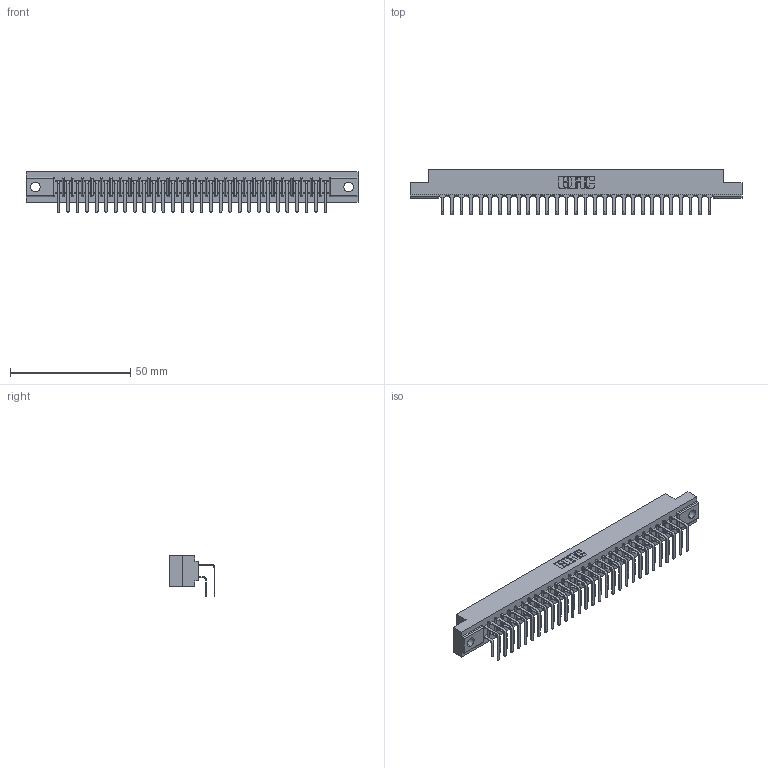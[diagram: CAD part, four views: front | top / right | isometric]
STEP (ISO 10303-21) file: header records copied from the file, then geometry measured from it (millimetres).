
FILE_DESCRIPTION (( 'STEP AP203' ), '1' );
FILE_NAME ('307-058-558-204.STEP', '2019-09-06T14:33:22', ( '' ), ( '' ), 'SwSTEP 2.0', 'SolidWorks 2016', '' );
FILE_SCHEMA (( 'CONFIG_CONTROL_DESIGN' ));
Length unit declared in the file: inch
Products named in the file (4): 307-290-001_558 559 - 1 (Single); 307-058-558-204; 307 Part_.156 Dia Mounting Holes; 307-290-001_558 - 2 (Single)
Assembly tree (59 placements, depth 2):
  307-058-558-204
    307 Part_.156 Dia Mounting Holes
    307-290-001_558 559 - 1 (Single)  x29
    307-290-001_558 - 2 (Single)  x29
Bounding box: 137.92 x 18.96 x 16.8 mm (x, y, z)
Volume: 14725.4 mm3; surface area: 19086.4 mm2
Topology: 59 solids, 59 shells, 3062 faces, 8595 edges, 5570 vertices
Faces by surface type: plane 1998, cylinder 1004, sphere 60
Entity records: 29257 total; most frequent: CARTESIAN_POINT 4797, ORIENTED_EDGE 4750, DIRECTION 4695, EDGE_CURVE 2375, LINE 1823, VECTOR 1823, VERTEX_POINT 1538, AXIS2_PLACEMENT_3D 1436
